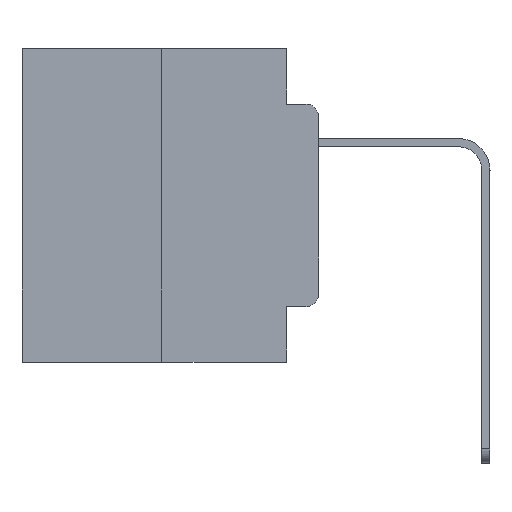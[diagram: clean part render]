
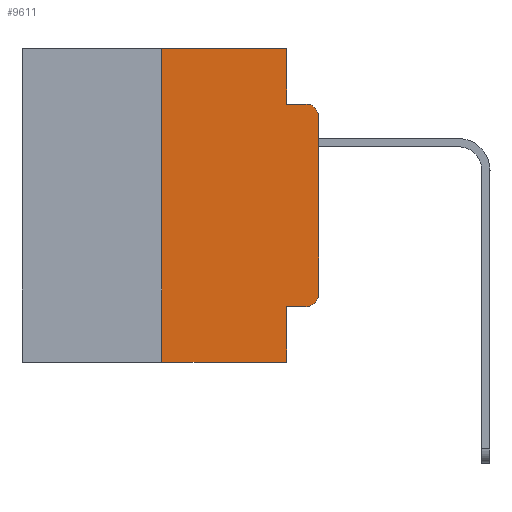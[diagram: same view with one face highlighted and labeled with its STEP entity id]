
A CAD part, left-side view. The second image highlights one B-rep face of the part: STEP entity #9611.
In plain terms, the highlighted planar face has unit normal (-1, 0, 0).
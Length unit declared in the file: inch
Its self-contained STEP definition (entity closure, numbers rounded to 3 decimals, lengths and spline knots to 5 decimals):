
#101 = LINE ( 'NONE', #22121, #727 ) ;
#359 = EDGE_LOOP ( 'NONE', ( #3321, #14869, #19659, #1441, #14088, #21880, #12993, #6641, #5015, #18391 ) ) ;
#727 = VECTOR ( 'NONE', #5829, 39.37008 ) ;
#811 = CARTESIAN_POINT ( 'NONE',  ( 0., 0.473, 0. ) ) ;
#1098 = EDGE_CURVE ( 'NONE', #14668, #3376, #20821, .T. ) ;
#1102 = FACE_OUTER_BOUND ( 'NONE', #359, .T. ) ;
#1441 = ORIENTED_EDGE ( 'NONE', *, *, #19293, .F. ) ;
#2102 = EDGE_CURVE ( 'NONE', #6238, #17706, #22675, .T. ) ;
#2843 = DIRECTION ( 'NONE',  ( -1., 0., 0. ) ) ;
#3321 = ORIENTED_EDGE ( 'NONE', *, *, #5026, .T. ) ;
#3376 = VERTEX_POINT ( 'NONE', #11864 ) ;
#3861 = VERTEX_POINT ( 'NONE', #21172 ) ;
#4418 = CARTESIAN_POINT ( 'NONE',  ( 0., 0.051, -0.0885 ) ) ;
#4515 = VECTOR ( 'NONE', #19866, 39.37008 ) ;
#4851 = VERTEX_POINT ( 'NONE', #18506 ) ;
#5015 = ORIENTED_EDGE ( 'NONE', *, *, #2102, .T. ) ;
#5026 = EDGE_CURVE ( 'NONE', #4851, #14668, #9138, .T. ) ;
#5457 = CARTESIAN_POINT ( 'NONE',  ( 0., 0., -0.1085 ) ) ;
#5483 = CARTESIAN_POINT ( 'NONE',  ( 0., 0.051, 0. ) ) ;
#5829 = DIRECTION ( 'NONE',  ( 0., -1., 0. ) ) ;
#6063 = PLANE ( 'NONE',  #17408 ) ;
#6238 = VERTEX_POINT ( 'NONE', #9243 ) ;
#6476 = VECTOR ( 'NONE', #22789, 39.37008 ) ;
#6641 = ORIENTED_EDGE ( 'NONE', *, *, #23930, .F. ) ;
#6878 = CARTESIAN_POINT ( 'NONE',  ( 0., 0.051, 0. ) ) ;
#8167 = DIRECTION ( 'NONE',  ( 1., 0., 0. ) ) ;
#8294 = LINE ( 'NONE', #20040, #22302 ) ;
#9138 = LINE ( 'NONE', #10856, #14724 ) ;
#9243 = CARTESIAN_POINT ( 'NONE',  ( 0., 0.051, -0.4115 ) ) ;
#9410 = VERTEX_POINT ( 'NONE', #25154 ) ;
#9611 = ADVANCED_FACE ( 'NONE', ( #1102 ), #6063, .F. ) ;
#10000 = CARTESIAN_POINT ( 'NONE',  ( 0., 0.473, 0. ) ) ;
#10206 = VECTOR ( 'NONE', #10985, 39.37008 ) ;
#10856 = CARTESIAN_POINT ( 'NONE',  ( 0., 0., 0. ) ) ;
#10876 = EDGE_CURVE ( 'NONE', #25531, #3376, #101, .T. ) ;
#10985 = DIRECTION ( 'NONE',  ( 0., 0., -1. ) ) ;
#11315 = AXIS2_PLACEMENT_3D ( 'NONE', #16629, #2843, #20796 ) ;
#11666 = CARTESIAN_POINT ( 'NONE',  ( 0., 0.02, -0.4115 ) ) ;
#11864 = CARTESIAN_POINT ( 'NONE',  ( 0., 0.02, -0.0885 ) ) ;
#12081 = EDGE_CURVE ( 'NONE', #9410, #3861, #12558, .T. ) ;
#12319 = CARTESIAN_POINT ( 'NONE',  ( 0., 0.051, -0.4115 ) ) ;
#12558 = LINE ( 'NONE', #20994, #25340 ) ;
#12993 = ORIENTED_EDGE ( 'NONE', *, *, #24770, .T. ) ;
#13153 = DIRECTION ( 'NONE',  ( 0., 0., -1. ) ) ;
#14088 = ORIENTED_EDGE ( 'NONE', *, *, #23326, .F. ) ;
#14668 = VERTEX_POINT ( 'NONE', #5457 ) ;
#14724 = VECTOR ( 'NONE', #15107, 39.37008 ) ;
#14869 = ORIENTED_EDGE ( 'NONE', *, *, #1098, .T. ) ;
#15107 = DIRECTION ( 'NONE',  ( 0., 0., 1. ) ) ;
#15338 = DIRECTION ( 'NONE',  ( 0., 0., 1. ) ) ;
#16138 = DIRECTION ( 'NONE',  ( 0., 0., -1. ) ) ;
#16146 = EDGE_CURVE ( 'NONE', #17706, #4851, #23551, .T. ) ;
#16601 = DIRECTION ( 'NONE',  ( 0., -1., 0. ) ) ;
#16629 = CARTESIAN_POINT ( 'NONE',  ( 0., 0.02, -0.3915 ) ) ;
#17081 = CARTESIAN_POINT ( 'NONE',  ( 0., 0.02, -0.1085 ) ) ;
#17380 = VECTOR ( 'NONE', #16601, 39.37008 ) ;
#17399 = LINE ( 'NONE', #811, #6476 ) ;
#17408 = AXIS2_PLACEMENT_3D ( 'NONE', #10000, #8167, #18076 ) ;
#17706 = VERTEX_POINT ( 'NONE', #11666 ) ;
#17975 = CARTESIAN_POINT ( 'NONE',  ( 0., 0.473, -0.5 ) ) ;
#18076 = DIRECTION ( 'NONE',  ( 0., 0., -1. ) ) ;
#18391 = ORIENTED_EDGE ( 'NONE', *, *, #16146, .T. ) ;
#18506 = CARTESIAN_POINT ( 'NONE',  ( 0., 0., -0.3915 ) ) ;
#19234 = DIRECTION ( 'NONE',  ( -1., 0., 0. ) ) ;
#19293 = EDGE_CURVE ( 'NONE', #22923, #25531, #8294, .T. ) ;
#19659 = ORIENTED_EDGE ( 'NONE', *, *, #10876, .F. ) ;
#19866 = DIRECTION ( 'NONE',  ( 0., -1., 0. ) ) ;
#20040 = CARTESIAN_POINT ( 'NONE',  ( 0., 0.051, 0. ) ) ;
#20796 = DIRECTION ( 'NONE',  ( 0., 0., -1. ) ) ;
#20821 = CIRCLE ( 'NONE', #22191, 0.02 ) ;
#20994 = CARTESIAN_POINT ( 'NONE',  ( 0., 0.25, 0. ) ) ;
#21172 = CARTESIAN_POINT ( 'NONE',  ( 0., 0.25, 0. ) ) ;
#21689 = LINE ( 'NONE', #17975, #4515 ) ;
#21730 = LINE ( 'NONE', #6878, #10206 ) ;
#21880 = ORIENTED_EDGE ( 'NONE', *, *, #12081, .F. ) ;
#22121 = CARTESIAN_POINT ( 'NONE',  ( 0., 0.051, -0.0885 ) ) ;
#22191 = AXIS2_PLACEMENT_3D ( 'NONE', #17081, #19234, #13153 ) ;
#22302 = VECTOR ( 'NONE', #16138, 39.37008 ) ;
#22434 = VERTEX_POINT ( 'NONE', #25696 ) ;
#22675 = LINE ( 'NONE', #12319, #17380 ) ;
#22789 = DIRECTION ( 'NONE',  ( 0., -1., 0. ) ) ;
#22923 = VERTEX_POINT ( 'NONE', #5483 ) ;
#23326 = EDGE_CURVE ( 'NONE', #3861, #22923, #17399, .T. ) ;
#23551 = CIRCLE ( 'NONE', #11315, 0.02 ) ;
#23930 = EDGE_CURVE ( 'NONE', #6238, #22434, #21730, .T. ) ;
#24770 = EDGE_CURVE ( 'NONE', #9410, #22434, #21689, .T. ) ;
#25154 = CARTESIAN_POINT ( 'NONE',  ( 0., 0.25, -0.5 ) ) ;
#25340 = VECTOR ( 'NONE', #15338, 39.37008 ) ;
#25531 = VERTEX_POINT ( 'NONE', #4418 ) ;
#25696 = CARTESIAN_POINT ( 'NONE',  ( 0., 0.051, -0.5 ) ) ;
